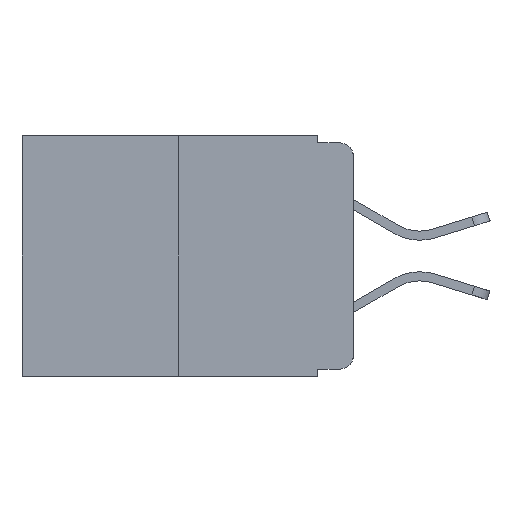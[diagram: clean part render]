
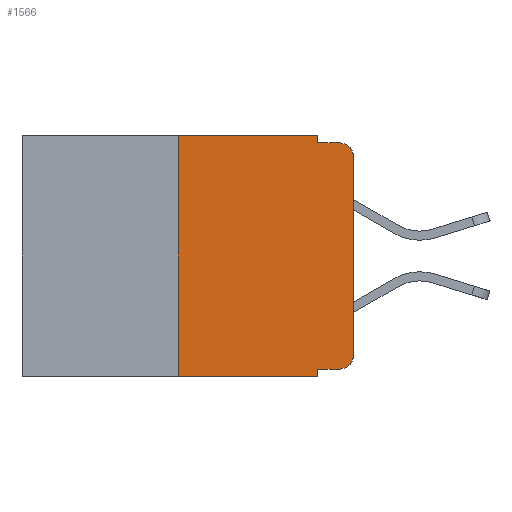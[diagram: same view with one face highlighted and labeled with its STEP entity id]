
A CAD part, left-side view. The second image highlights one B-rep face of the part: STEP entity #1566.
In plain terms, the highlighted planar face has unit normal (-1, 0, 0).
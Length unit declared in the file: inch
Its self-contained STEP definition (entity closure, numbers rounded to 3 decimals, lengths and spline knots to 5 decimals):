
#68 = EDGE_CURVE ( 'NONE', #9190, #11777, #4943, .T. ) ;
#128 = CARTESIAN_POINT ( 'NONE',  ( 0., 0.051, -0.343 ) ) ;
#195 = EDGE_CURVE ( 'NONE', #8919, #7193, #13068, .T. ) ;
#504 = DIRECTION ( 'NONE',  ( 0., -1., 0. ) ) ;
#512 = DIRECTION ( 'NONE',  ( 0., -1., 0. ) ) ;
#786 = EDGE_CURVE ( 'NONE', #16315, #9190, #4441, .T. ) ;
#897 = DIRECTION ( 'NONE',  ( 1., 0., 0. ) ) ;
#1105 = CARTESIAN_POINT ( 'NONE',  ( 0., 0.25, -0.343 ) ) ;
#1566 = ADVANCED_FACE ( 'NONE', ( #2230 ), #6969, .F. ) ;
#1941 = EDGE_CURVE ( 'NONE', #7193, #18489, #3162, .T. ) ;
#2053 = CARTESIAN_POINT ( 'NONE',  ( 0., 0., -0.03 ) ) ;
#2230 = FACE_OUTER_BOUND ( 'NONE', #8411, .T. ) ;
#2554 = EDGE_CURVE ( 'NONE', #16315, #11328, #15415, .T. ) ;
#2606 = CARTESIAN_POINT ( 'NONE',  ( 0., 0.051, 0. ) ) ;
#2665 = AXIS2_PLACEMENT_3D ( 'NONE', #11583, #5523, #13170 ) ;
#3162 = LINE ( 'NONE', #11166, #3645 ) ;
#3416 = LINE ( 'NONE', #18945, #15468 ) ;
#3645 = VECTOR ( 'NONE', #12939, 39.37008 ) ;
#3740 = DIRECTION ( 'NONE',  ( 0., 0., 1. ) ) ;
#4043 = EDGE_CURVE ( 'NONE', #17371, #7253, #11423, .T. ) ;
#4135 = ORIENTED_EDGE ( 'NONE', *, *, #7212, .F. ) ;
#4356 = DIRECTION ( 'NONE',  ( 0., 0., -1. ) ) ;
#4441 = LINE ( 'NONE', #14453, #8124 ) ;
#4754 = CARTESIAN_POINT ( 'NONE',  ( 0., 0.473, -0.343 ) ) ;
#4943 = LINE ( 'NONE', #17675, #15981 ) ;
#5324 = VECTOR ( 'NONE', #18737, 39.37008 ) ;
#5523 = DIRECTION ( 'NONE',  ( -1., 0., 0. ) ) ;
#5891 = LINE ( 'NONE', #2606, #13786 ) ;
#6066 = ORIENTED_EDGE ( 'NONE', *, *, #786, .F. ) ;
#6173 = CARTESIAN_POINT ( 'NONE',  ( 0., 0.02, -0.03 ) ) ;
#6225 = ORIENTED_EDGE ( 'NONE', *, *, #10785, .T. ) ;
#6442 = ORIENTED_EDGE ( 'NONE', *, *, #1941, .T. ) ;
#6969 = PLANE ( 'NONE',  #11224 ) ;
#7064 = ORIENTED_EDGE ( 'NONE', *, *, #8937, .F. ) ;
#7193 = VERTEX_POINT ( 'NONE', #10549 ) ;
#7212 = EDGE_CURVE ( 'NONE', #11777, #17371, #5891, .T. ) ;
#7241 = VECTOR ( 'NONE', #17126, 39.37008 ) ;
#7253 = VERTEX_POINT ( 'NONE', #20186 ) ;
#8065 = ORIENTED_EDGE ( 'NONE', *, *, #4043, .F. ) ;
#8124 = VECTOR ( 'NONE', #3740, 39.37008 ) ;
#8411 = EDGE_LOOP ( 'NONE', ( #6442, #11368, #8065, #4135, #20268, #6066, #19423, #7064, #6225, #13140 ) ) ;
#8503 = LINE ( 'NONE', #16246, #20015 ) ;
#8919 = VERTEX_POINT ( 'NONE', #10760 ) ;
#8937 = EDGE_CURVE ( 'NONE', #11674, #11328, #3416, .T. ) ;
#9190 = VERTEX_POINT ( 'NONE', #10061 ) ;
#10061 = CARTESIAN_POINT ( 'NONE',  ( 0., 0.25, 0. ) ) ;
#10549 = CARTESIAN_POINT ( 'NONE',  ( 0., 0., -0.313 ) ) ;
#10760 = CARTESIAN_POINT ( 'NONE',  ( 0., 0.02, -0.333 ) ) ;
#10785 = EDGE_CURVE ( 'NONE', #11674, #8919, #8503, .T. ) ;
#11166 = CARTESIAN_POINT ( 'NONE',  ( 0., 0., 0. ) ) ;
#11224 = AXIS2_PLACEMENT_3D ( 'NONE', #11935, #897, #14813 ) ;
#11328 = VERTEX_POINT ( 'NONE', #128 ) ;
#11368 = ORIENTED_EDGE ( 'NONE', *, *, #12868, .T. ) ;
#11423 = LINE ( 'NONE', #13997, #7241 ) ;
#11583 = CARTESIAN_POINT ( 'NONE',  ( 0., 0.02, -0.313 ) ) ;
#11674 = VERTEX_POINT ( 'NONE', #12225 ) ;
#11777 = VERTEX_POINT ( 'NONE', #20014 ) ;
#11935 = CARTESIAN_POINT ( 'NONE',  ( 0., 0.473, 0. ) ) ;
#12225 = CARTESIAN_POINT ( 'NONE',  ( 0., 0.051, -0.333 ) ) ;
#12868 = EDGE_CURVE ( 'NONE', #18489, #7253, #13947, .T. ) ;
#12939 = DIRECTION ( 'NONE',  ( 0., 0., 1. ) ) ;
#13068 = CIRCLE ( 'NONE', #2665, 0.02 ) ;
#13140 = ORIENTED_EDGE ( 'NONE', *, *, #195, .T. ) ;
#13170 = DIRECTION ( 'NONE',  ( 0., 0., -1. ) ) ;
#13475 = CARTESIAN_POINT ( 'NONE',  ( 0., 0.051, -0.01 ) ) ;
#13786 = VECTOR ( 'NONE', #4356, 39.37008 ) ;
#13947 = CIRCLE ( 'NONE', #15056, 0.02 ) ;
#13997 = CARTESIAN_POINT ( 'NONE',  ( 0., 0.051, -0.01 ) ) ;
#14453 = CARTESIAN_POINT ( 'NONE',  ( 0., 0.25, 0. ) ) ;
#14813 = DIRECTION ( 'NONE',  ( 0., 0., -1. ) ) ;
#15056 = AXIS2_PLACEMENT_3D ( 'NONE', #6173, #17296, #17434 ) ;
#15415 = LINE ( 'NONE', #4754, #5324 ) ;
#15468 = VECTOR ( 'NONE', #17647, 39.37008 ) ;
#15981 = VECTOR ( 'NONE', #504, 39.37008 ) ;
#16246 = CARTESIAN_POINT ( 'NONE',  ( 0., 0.051, -0.333 ) ) ;
#16315 = VERTEX_POINT ( 'NONE', #1105 ) ;
#17126 = DIRECTION ( 'NONE',  ( 0., -1., 0. ) ) ;
#17296 = DIRECTION ( 'NONE',  ( -1., 0., 0. ) ) ;
#17371 = VERTEX_POINT ( 'NONE', #13475 ) ;
#17434 = DIRECTION ( 'NONE',  ( 0., 0., -1. ) ) ;
#17647 = DIRECTION ( 'NONE',  ( 0., 0., -1. ) ) ;
#17675 = CARTESIAN_POINT ( 'NONE',  ( 0., 0.473, 0. ) ) ;
#18489 = VERTEX_POINT ( 'NONE', #2053 ) ;
#18737 = DIRECTION ( 'NONE',  ( 0., -1., 0. ) ) ;
#18945 = CARTESIAN_POINT ( 'NONE',  ( 0., 0.051, 0. ) ) ;
#19423 = ORIENTED_EDGE ( 'NONE', *, *, #2554, .T. ) ;
#20014 = CARTESIAN_POINT ( 'NONE',  ( 0., 0.051, 0. ) ) ;
#20015 = VECTOR ( 'NONE', #512, 39.37008 ) ;
#20186 = CARTESIAN_POINT ( 'NONE',  ( 0., 0.02, -0.01 ) ) ;
#20268 = ORIENTED_EDGE ( 'NONE', *, *, #68, .F. ) ;
